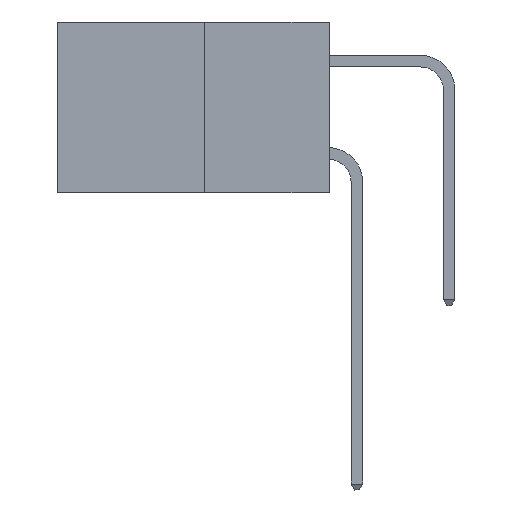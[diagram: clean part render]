
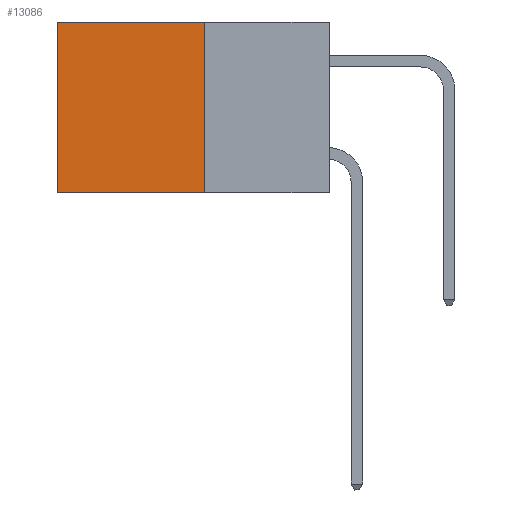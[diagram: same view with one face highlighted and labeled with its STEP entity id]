
A CAD part, left-side view. The second image highlights one B-rep face of the part: STEP entity #13086.
In plain terms, the highlighted planar face has unit normal (-1, 0, 0).
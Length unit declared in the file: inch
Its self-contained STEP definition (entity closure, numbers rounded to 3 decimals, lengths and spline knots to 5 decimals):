
#495 = ORIENTED_EDGE ( 'NONE', *, *, #8030, .F. ) ;
#815 = LINE ( 'NONE', #11965, #14329 ) ;
#846 = CARTESIAN_POINT ( 'NONE',  ( 0.277, 0.27, 0. ) ) ;
#902 = DIRECTION ( 'NONE',  ( 0., 0., -1. ) ) ;
#970 = DIRECTION ( 'NONE',  ( 0., 1., 0. ) ) ;
#1301 = VECTOR ( 'NONE', #970, 39.37008 ) ;
#1508 = CARTESIAN_POINT ( 'NONE',  ( 0.277, 0.27, 0. ) ) ;
#1617 = CARTESIAN_POINT ( 'NONE',  ( 0.277, 0.27, -0.37 ) ) ;
#1813 = VECTOR ( 'NONE', #902, 39.37008 ) ;
#1820 = DIRECTION ( 'NONE',  ( 0., 1., 0. ) ) ;
#2117 = VECTOR ( 'NONE', #1820, 39.37008 ) ;
#2136 = CARTESIAN_POINT ( 'NONE',  ( 0.277, 0.59, 0. ) ) ;
#2186 = CARTESIAN_POINT ( 'NONE',  ( 0.277, 0.59, -0.37 ) ) ;
#2283 = VERTEX_POINT ( 'NONE', #2136 ) ;
#3628 = EDGE_CURVE ( 'NONE', #12676, #11344, #815, .T. ) ;
#6903 = VERTEX_POINT ( 'NONE', #7389 ) ;
#6965 = EDGE_CURVE ( 'NONE', #12676, #2283, #15217, .T. ) ;
#7389 = CARTESIAN_POINT ( 'NONE',  ( 0.277, 0.59, -0.37 ) ) ;
#7546 = DIRECTION ( 'NONE',  ( 1., 0., 0. ) ) ;
#7932 = ORIENTED_EDGE ( 'NONE', *, *, #3628, .F. ) ;
#8030 = EDGE_CURVE ( 'NONE', #11344, #6903, #9064, .T. ) ;
#8764 = LINE ( 'NONE', #2186, #1813 ) ;
#9064 = LINE ( 'NONE', #12217, #2117 ) ;
#10037 = ORIENTED_EDGE ( 'NONE', *, *, #15379, .T. ) ;
#11344 = VERTEX_POINT ( 'NONE', #1617 ) ;
#11382 = DIRECTION ( 'NONE',  ( 0., 0., -1. ) ) ;
#11965 = CARTESIAN_POINT ( 'NONE',  ( 0.277, 0.27, -0.37 ) ) ;
#12200 = ORIENTED_EDGE ( 'NONE', *, *, #6965, .T. ) ;
#12217 = CARTESIAN_POINT ( 'NONE',  ( 0.277, 0.27, -0.37 ) ) ;
#12638 = PLANE ( 'NONE',  #16087 ) ;
#12676 = VERTEX_POINT ( 'NONE', #1508 ) ;
#13086 = ADVANCED_FACE ( 'NONE', ( #15155 ), #12638, .F. ) ;
#13925 = EDGE_LOOP ( 'NONE', ( #10037, #495, #7932, #12200 ) ) ;
#14329 = VECTOR ( 'NONE', #11382, 39.37008 ) ;
#15155 = FACE_OUTER_BOUND ( 'NONE', #13925, .T. ) ;
#15217 = LINE ( 'NONE', #846, #1301 ) ;
#15332 = CARTESIAN_POINT ( 'NONE',  ( 0.277, 0.27, -0.37 ) ) ;
#15379 = EDGE_CURVE ( 'NONE', #2283, #6903, #8764, .T. ) ;
#16087 = AXIS2_PLACEMENT_3D ( 'NONE', #15332, #7546, #16666 ) ;
#16666 = DIRECTION ( 'NONE',  ( 0., 0., -1. ) ) ;
